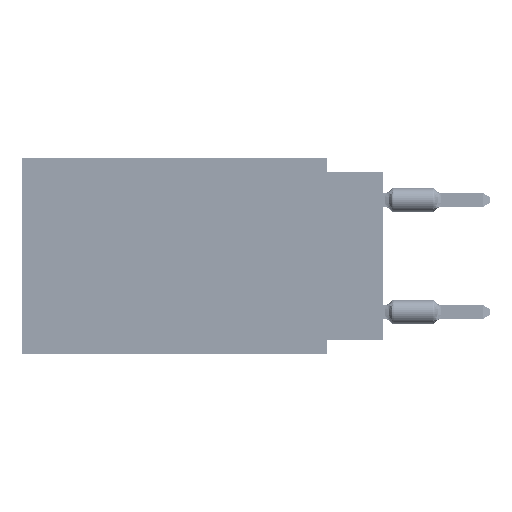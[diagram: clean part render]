
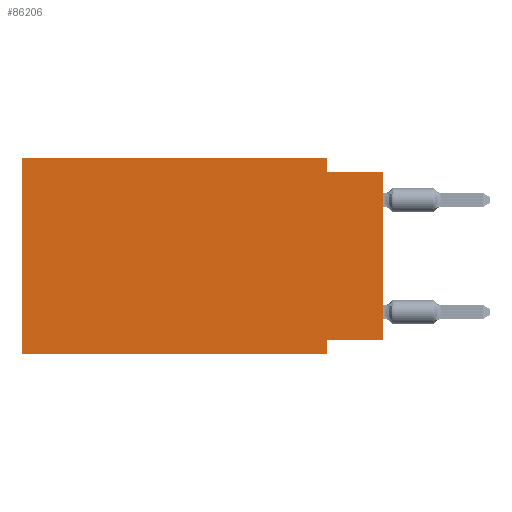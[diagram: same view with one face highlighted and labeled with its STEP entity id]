
A CAD part, left-side view. The second image highlights one B-rep face of the part: STEP entity #86206.
In plain terms, the highlighted planar face has unit normal (-1, 0, 0).
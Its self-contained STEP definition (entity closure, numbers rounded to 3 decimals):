
#253 = VECTOR ( 'NONE', #21568, 1000. ) ;
#619 = FACE_OUTER_BOUND ( 'NONE', #90395, .T. ) ;
#993 = VECTOR ( 'NONE', #46216, 1000. ) ;
#3148 = CARTESIAN_POINT ( 'NONE',  ( 0., 2.54, -8.89 ) ) ;
#5451 = CARTESIAN_POINT ( 'NONE',  ( 0., 0., 0. ) ) ;
#7023 = CARTESIAN_POINT ( 'NONE',  ( 0., 0., -8.255 ) ) ;
#8210 = DIRECTION ( 'NONE',  ( 0., 1., 0. ) ) ;
#9120 = ORIENTED_EDGE ( 'NONE', *, *, #11109, .F. ) ;
#9216 = EDGE_CURVE ( 'NONE', #92756, #47017, #31645, .T. ) ;
#10589 = CARTESIAN_POINT ( 'NONE',  ( 0., 0., -0.635 ) ) ;
#11109 = EDGE_CURVE ( 'NONE', #110750, #87082, #64077, .T. ) ;
#12312 = LINE ( 'NONE', #30738, #35037 ) ;
#16317 = ORIENTED_EDGE ( 'NONE', *, *, #9216, .F. ) ;
#19059 = EDGE_CURVE ( 'NONE', #95062, #110750, #93118, .T. ) ;
#19508 = DIRECTION ( 'NONE',  ( 0., -1., 0. ) ) ;
#21568 = DIRECTION ( 'NONE',  ( 0., 0., -1. ) ) ;
#21573 = VERTEX_POINT ( 'NONE', #38075 ) ;
#23619 = ORIENTED_EDGE ( 'NONE', *, *, #30498, .T. ) ;
#24290 = LINE ( 'NONE', #7023, #43041 ) ;
#26831 = ORIENTED_EDGE ( 'NONE', *, *, #55443, .T. ) ;
#28955 = LINE ( 'NONE', #63434, #75473 ) ;
#30498 = EDGE_CURVE ( 'NONE', #21573, #87082, #96323, .T. ) ;
#30738 = CARTESIAN_POINT ( 'NONE',  ( 0., 16.383, -8.89 ) ) ;
#31115 = VECTOR ( 'NONE', #19508, 1000. ) ;
#31645 = LINE ( 'NONE', #3148, #253 ) ;
#35037 = VECTOR ( 'NONE', #93132, 1000. ) ;
#38075 = CARTESIAN_POINT ( 'NONE',  ( 0., 0., -8.255 ) ) ;
#43041 = VECTOR ( 'NONE', #8210, 1000. ) ;
#46216 = DIRECTION ( 'NONE',  ( 0., 0., -1. ) ) ;
#47017 = VERTEX_POINT ( 'NONE', #56151 ) ;
#51126 = CARTESIAN_POINT ( 'NONE',  ( 0., 16.383, 0. ) ) ;
#52279 = ORIENTED_EDGE ( 'NONE', *, *, #76631, .F. ) ;
#52727 = VERTEX_POINT ( 'NONE', #91975 ) ;
#53291 = CARTESIAN_POINT ( 'NONE',  ( 0., 2.54, -0.635 ) ) ;
#53981 = DIRECTION ( 'NONE',  ( 0., -1., 0. ) ) ;
#54433 = CARTESIAN_POINT ( 'NONE',  ( 0., 0., -0.635 ) ) ;
#55065 = ORIENTED_EDGE ( 'NONE', *, *, #19059, .F. ) ;
#55443 = EDGE_CURVE ( 'NONE', #52727, #47017, #12312, .T. ) ;
#56151 = CARTESIAN_POINT ( 'NONE',  ( 0., 2.54, -8.89 ) ) ;
#58980 = CARTESIAN_POINT ( 'NONE',  ( 0., 2.54, -8.255 ) ) ;
#61258 = DIRECTION ( 'NONE',  ( 0., 0., -1. ) ) ;
#63132 = ORIENTED_EDGE ( 'NONE', *, *, #70012, .F. ) ;
#63434 = CARTESIAN_POINT ( 'NONE',  ( 0., 16.383, 0. ) ) ;
#64077 = LINE ( 'NONE', #10589, #101294 ) ;
#64639 = CARTESIAN_POINT ( 'NONE',  ( 0., 2.54, 0. ) ) ;
#70012 = EDGE_CURVE ( 'NONE', #76205, #95062, #83662, .T. ) ;
#70180 = PLANE ( 'NONE',  #93178 ) ;
#72660 = VECTOR ( 'NONE', #104659, 1000. ) ;
#74131 = EDGE_CURVE ( 'NONE', #21573, #92756, #24290, .T. ) ;
#75473 = VECTOR ( 'NONE', #99630, 1000. ) ;
#76205 = VERTEX_POINT ( 'NONE', #51126 ) ;
#76631 = EDGE_CURVE ( 'NONE', #52727, #76205, #28955, .T. ) ;
#83662 = LINE ( 'NONE', #101455, #31115 ) ;
#86206 = ADVANCED_FACE ( 'NONE', ( #619 ), #70180, .F. ) ;
#87082 = VERTEX_POINT ( 'NONE', #54433 ) ;
#90395 = EDGE_LOOP ( 'NONE', ( #23619, #9120, #55065, #63132, #52279, #26831, #16317, #98557 ) ) ;
#91975 = CARTESIAN_POINT ( 'NONE',  ( 0., 16.383, -8.89 ) ) ;
#92756 = VERTEX_POINT ( 'NONE', #58980 ) ;
#93118 = LINE ( 'NONE', #64639, #993 ) ;
#93132 = DIRECTION ( 'NONE',  ( 0., -1., 0. ) ) ;
#93178 = AXIS2_PLACEMENT_3D ( 'NONE', #106394, #107590, #61258 ) ;
#95062 = VERTEX_POINT ( 'NONE', #99503 ) ;
#96323 = LINE ( 'NONE', #5451, #72660 ) ;
#98557 = ORIENTED_EDGE ( 'NONE', *, *, #74131, .F. ) ;
#99503 = CARTESIAN_POINT ( 'NONE',  ( 0., 2.54, 0. ) ) ;
#99630 = DIRECTION ( 'NONE',  ( 0., 0., 1. ) ) ;
#101294 = VECTOR ( 'NONE', #53981, 1000. ) ;
#101455 = CARTESIAN_POINT ( 'NONE',  ( 0., 16.383, 0. ) ) ;
#104659 = DIRECTION ( 'NONE',  ( 0., 0., 1. ) ) ;
#106394 = CARTESIAN_POINT ( 'NONE',  ( 0., 16.383, 0. ) ) ;
#107590 = DIRECTION ( 'NONE',  ( 1., 0., 0. ) ) ;
#110750 = VERTEX_POINT ( 'NONE', #53291 ) ;
